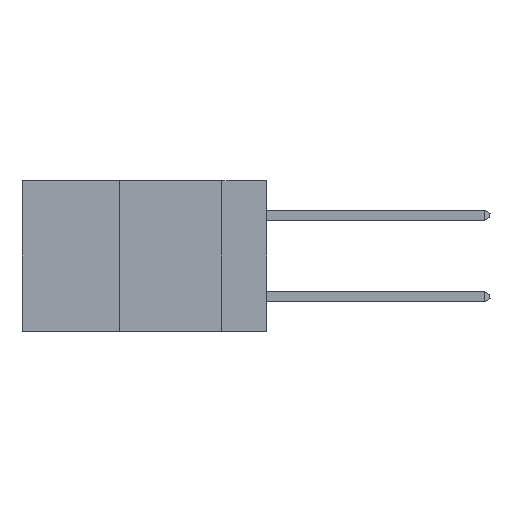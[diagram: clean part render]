
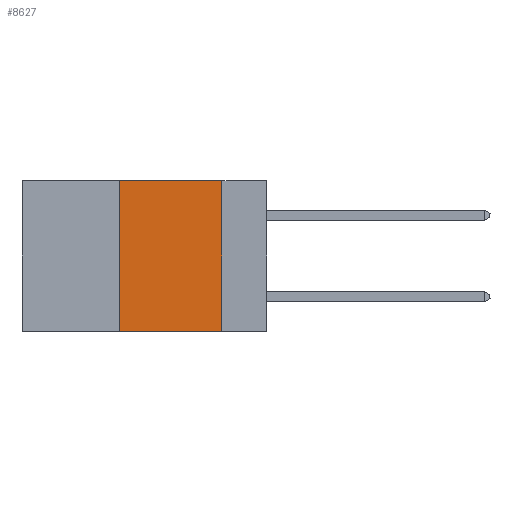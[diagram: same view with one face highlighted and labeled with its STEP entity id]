
A CAD part, left-side view. The second image highlights one B-rep face of the part: STEP entity #8627.
In plain terms, the highlighted planar face has unit normal (-1, 0, 0).
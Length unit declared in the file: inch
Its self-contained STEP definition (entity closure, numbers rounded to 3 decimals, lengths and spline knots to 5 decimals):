
#554 = CARTESIAN_POINT ( 'NONE',  ( 0., 0.6, -0.37 ) ) ;
#559 = AXIS2_PLACEMENT_3D ( 'NONE', #10529, #8775, #2316 ) ;
#593 = EDGE_CURVE ( 'NONE', #11801, #7251, #13041, .T. ) ;
#1172 = LINE ( 'NONE', #554, #12122 ) ;
#1211 = CARTESIAN_POINT ( 'NONE',  ( 0., 0.36, -0.37 ) ) ;
#1436 = ORIENTED_EDGE ( 'NONE', *, *, #593, .F. ) ;
#2192 = CARTESIAN_POINT ( 'NONE',  ( 0., 0.11, -0.37 ) ) ;
#2316 = DIRECTION ( 'NONE',  ( 0., 0., -1. ) ) ;
#2344 = DIRECTION ( 'NONE',  ( 0., -1., 0. ) ) ;
#2543 = FACE_OUTER_BOUND ( 'NONE', #8731, .T. ) ;
#2748 = CARTESIAN_POINT ( 'NONE',  ( 0., 0.36, 0. ) ) ;
#2754 = ORIENTED_EDGE ( 'NONE', *, *, #13759, .T. ) ;
#4062 = EDGE_CURVE ( 'NONE', #12131, #11801, #12442, .T. ) ;
#6078 = DIRECTION ( 'NONE',  ( 0., 0., -1. ) ) ;
#6236 = PLANE ( 'NONE',  #559 ) ;
#7251 = VERTEX_POINT ( 'NONE', #10408 ) ;
#7296 = VECTOR ( 'NONE', #10231, 39.37008 ) ;
#7757 = LINE ( 'NONE', #10445, #9499 ) ;
#8460 = DIRECTION ( 'NONE',  ( 0., -1., 0. ) ) ;
#8627 = ADVANCED_FACE ( 'NONE', ( #2543 ), #6236, .F. ) ;
#8731 = EDGE_LOOP ( 'NONE', ( #12938, #1436, #10599, #2754 ) ) ;
#8775 = DIRECTION ( 'NONE',  ( 1., 0., 0. ) ) ;
#9062 = CARTESIAN_POINT ( 'NONE',  ( 0., 0.6, 0. ) ) ;
#9098 = CARTESIAN_POINT ( 'NONE',  ( 0., 0.36, 0. ) ) ;
#9185 = VERTEX_POINT ( 'NONE', #2192 ) ;
#9475 = EDGE_CURVE ( 'NONE', #7251, #9185, #7757, .T. ) ;
#9499 = VECTOR ( 'NONE', #6078, 39.37008 ) ;
#10231 = DIRECTION ( 'NONE',  ( 0., 0., 1. ) ) ;
#10408 = CARTESIAN_POINT ( 'NONE',  ( 0., 0.11, 0. ) ) ;
#10445 = CARTESIAN_POINT ( 'NONE',  ( 0., 0.11, 0. ) ) ;
#10529 = CARTESIAN_POINT ( 'NONE',  ( 0., 0.6, 0. ) ) ;
#10599 = ORIENTED_EDGE ( 'NONE', *, *, #4062, .F. ) ;
#11801 = VERTEX_POINT ( 'NONE', #9098 ) ;
#12122 = VECTOR ( 'NONE', #8460, 39.37008 ) ;
#12131 = VERTEX_POINT ( 'NONE', #1211 ) ;
#12442 = LINE ( 'NONE', #2748, #7296 ) ;
#12938 = ORIENTED_EDGE ( 'NONE', *, *, #9475, .F. ) ;
#13041 = LINE ( 'NONE', #9062, #13903 ) ;
#13759 = EDGE_CURVE ( 'NONE', #12131, #9185, #1172, .T. ) ;
#13903 = VECTOR ( 'NONE', #2344, 39.37008 ) ;
